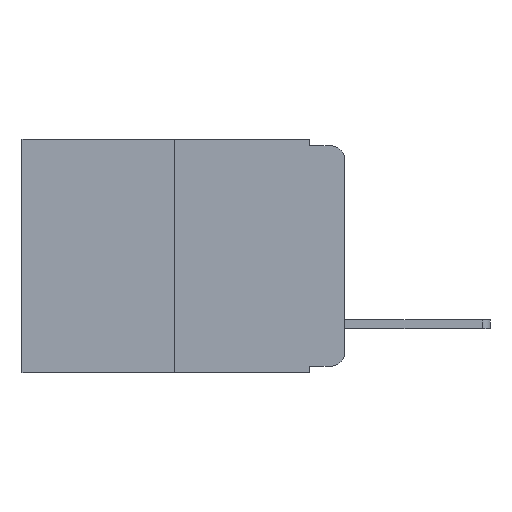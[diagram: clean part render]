
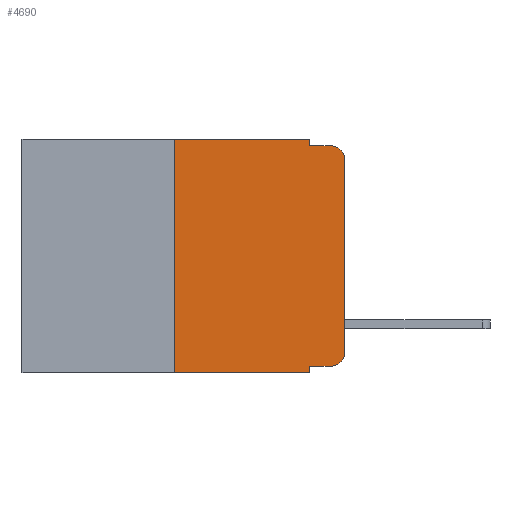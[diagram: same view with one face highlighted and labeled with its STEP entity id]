
A CAD part, left-side view. The second image highlights one B-rep face of the part: STEP entity #4690.
In plain terms, the highlighted planar face has unit normal (-1, 0, 0).
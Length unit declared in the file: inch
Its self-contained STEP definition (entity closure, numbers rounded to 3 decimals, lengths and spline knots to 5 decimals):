
#315 = LINE ( 'NONE', #5412, #9951 ) ;
#728 = LINE ( 'NONE', #15327, #10292 ) ;
#776 = EDGE_CURVE ( 'NONE', #5272, #4673, #3199, .T. ) ;
#1044 = CARTESIAN_POINT ( 'NONE',  ( 0., 0.02, -0.333 ) ) ;
#1351 = LINE ( 'NONE', #7830, #10848 ) ;
#1625 = VECTOR ( 'NONE', #12770, 39.37008 ) ;
#1779 = EDGE_CURVE ( 'NONE', #7824, #7643, #2334, .T. ) ;
#1856 = LINE ( 'NONE', #3908, #11316 ) ;
#2014 = LINE ( 'NONE', #4101, #14632 ) ;
#2041 = DIRECTION ( 'NONE',  ( 0., 0., -1. ) ) ;
#2334 = LINE ( 'NONE', #2532, #8533 ) ;
#2532 = CARTESIAN_POINT ( 'NONE',  ( 0., 0.051, 0. ) ) ;
#2682 = EDGE_CURVE ( 'NONE', #7643, #8608, #2014, .T. ) ;
#2789 = VECTOR ( 'NONE', #10653, 39.37008 ) ;
#3029 = CARTESIAN_POINT ( 'NONE',  ( 0., 0.051, -0.333 ) ) ;
#3199 = LINE ( 'NONE', #14779, #2789 ) ;
#3526 = CARTESIAN_POINT ( 'NONE',  ( 0., 0., -0.03 ) ) ;
#3545 = ORIENTED_EDGE ( 'NONE', *, *, #15193, .F. ) ;
#3546 = EDGE_CURVE ( 'NONE', #5407, #8608, #6172, .T. ) ;
#3800 = DIRECTION ( 'NONE',  ( 0., 0., -1. ) ) ;
#3908 = CARTESIAN_POINT ( 'NONE',  ( 0., 0., 0. ) ) ;
#3928 = ORIENTED_EDGE ( 'NONE', *, *, #12009, .T. ) ;
#4101 = CARTESIAN_POINT ( 'NONE',  ( 0., 0.051, -0.01 ) ) ;
#4673 = VERTEX_POINT ( 'NONE', #14808 ) ;
#4690 = ADVANCED_FACE ( 'NONE', ( #9327 ), #10798, .F. ) ;
#5159 = AXIS2_PLACEMENT_3D ( 'NONE', #8337, #7938, #9283 ) ;
#5178 = DIRECTION ( 'NONE',  ( -1., 0., 0. ) ) ;
#5272 = VERTEX_POINT ( 'NONE', #7022 ) ;
#5379 = DIRECTION ( 'NONE',  ( 0., 0., 1. ) ) ;
#5407 = VERTEX_POINT ( 'NONE', #3526 ) ;
#5412 = CARTESIAN_POINT ( 'NONE',  ( 0., 0.051, 0. ) ) ;
#5427 = LINE ( 'NONE', #3029, #1625 ) ;
#6172 = CIRCLE ( 'NONE', #14734, 0.02 ) ;
#6313 = CARTESIAN_POINT ( 'NONE',  ( 0., 0.25, 0. ) ) ;
#6361 = VERTEX_POINT ( 'NONE', #13818 ) ;
#6376 = DIRECTION ( 'NONE',  ( -1., 0., 0. ) ) ;
#6871 = ORIENTED_EDGE ( 'NONE', *, *, #12803, .T. ) ;
#6898 = EDGE_CURVE ( 'NONE', #11476, #5407, #1856, .T. ) ;
#7022 = CARTESIAN_POINT ( 'NONE',  ( 0., 0.25, -0.343 ) ) ;
#7643 = VERTEX_POINT ( 'NONE', #12909 ) ;
#7652 = CARTESIAN_POINT ( 'NONE',  ( 0., 0.02, -0.01 ) ) ;
#7824 = VERTEX_POINT ( 'NONE', #12019 ) ;
#7830 = CARTESIAN_POINT ( 'NONE',  ( 0., 0.473, 0. ) ) ;
#7938 = DIRECTION ( 'NONE',  ( 1., 0., 0. ) ) ;
#8125 = AXIS2_PLACEMENT_3D ( 'NONE', #12430, #5178, #13615 ) ;
#8337 = CARTESIAN_POINT ( 'NONE',  ( 0., 0.473, 0. ) ) ;
#8517 = ORIENTED_EDGE ( 'NONE', *, *, #6898, .T. ) ;
#8533 = VECTOR ( 'NONE', #2041, 39.37008 ) ;
#8608 = VERTEX_POINT ( 'NONE', #7652 ) ;
#9005 = DIRECTION ( 'NONE',  ( 0., -1., 0. ) ) ;
#9283 = DIRECTION ( 'NONE',  ( 0., 0., -1. ) ) ;
#9327 = FACE_OUTER_BOUND ( 'NONE', #12348, .T. ) ;
#9887 = CARTESIAN_POINT ( 'NONE',  ( 0., 0., -0.313 ) ) ;
#9951 = VECTOR ( 'NONE', #15038, 39.37008 ) ;
#10292 = VECTOR ( 'NONE', #14023, 39.37008 ) ;
#10653 = DIRECTION ( 'NONE',  ( 0., -1., 0. ) ) ;
#10798 = PLANE ( 'NONE',  #5159 ) ;
#10848 = VECTOR ( 'NONE', #9005, 39.37008 ) ;
#11316 = VECTOR ( 'NONE', #5379, 39.37008 ) ;
#11476 = VERTEX_POINT ( 'NONE', #9887 ) ;
#12009 = EDGE_CURVE ( 'NONE', #12508, #11476, #13711, .T. ) ;
#12019 = CARTESIAN_POINT ( 'NONE',  ( 0., 0.051, 0. ) ) ;
#12103 = ORIENTED_EDGE ( 'NONE', *, *, #2682, .F. ) ;
#12348 = EDGE_LOOP ( 'NONE', ( #8517, #14897, #12103, #15265, #12478, #15616, #12852, #3545, #6871, #3928 ) ) ;
#12430 = CARTESIAN_POINT ( 'NONE',  ( 0., 0.02, -0.313 ) ) ;
#12478 = ORIENTED_EDGE ( 'NONE', *, *, #14332, .F. ) ;
#12508 = VERTEX_POINT ( 'NONE', #1044 ) ;
#12770 = DIRECTION ( 'NONE',  ( 0., -1., 0. ) ) ;
#12803 = EDGE_CURVE ( 'NONE', #6361, #12508, #5427, .T. ) ;
#12852 = ORIENTED_EDGE ( 'NONE', *, *, #776, .T. ) ;
#12909 = CARTESIAN_POINT ( 'NONE',  ( 0., 0.051, -0.01 ) ) ;
#13558 = CARTESIAN_POINT ( 'NONE',  ( 0., 0.02, -0.03 ) ) ;
#13615 = DIRECTION ( 'NONE',  ( 0., 0., -1. ) ) ;
#13619 = VERTEX_POINT ( 'NONE', #6313 ) ;
#13711 = CIRCLE ( 'NONE', #8125, 0.02 ) ;
#13818 = CARTESIAN_POINT ( 'NONE',  ( 0., 0.051, -0.333 ) ) ;
#14023 = DIRECTION ( 'NONE',  ( 0., 0., 1. ) ) ;
#14332 = EDGE_CURVE ( 'NONE', #13619, #7824, #1351, .T. ) ;
#14632 = VECTOR ( 'NONE', #14718, 39.37008 ) ;
#14718 = DIRECTION ( 'NONE',  ( 0., -1., 0. ) ) ;
#14734 = AXIS2_PLACEMENT_3D ( 'NONE', #13558, #6376, #3800 ) ;
#14779 = CARTESIAN_POINT ( 'NONE',  ( 0., 0.473, -0.343 ) ) ;
#14808 = CARTESIAN_POINT ( 'NONE',  ( 0., 0.051, -0.343 ) ) ;
#14897 = ORIENTED_EDGE ( 'NONE', *, *, #3546, .T. ) ;
#15038 = DIRECTION ( 'NONE',  ( 0., 0., -1. ) ) ;
#15193 = EDGE_CURVE ( 'NONE', #6361, #4673, #315, .T. ) ;
#15265 = ORIENTED_EDGE ( 'NONE', *, *, #1779, .F. ) ;
#15327 = CARTESIAN_POINT ( 'NONE',  ( 0., 0.25, 0. ) ) ;
#15616 = ORIENTED_EDGE ( 'NONE', *, *, #15964, .F. ) ;
#15964 = EDGE_CURVE ( 'NONE', #5272, #13619, #728, .T. ) ;
